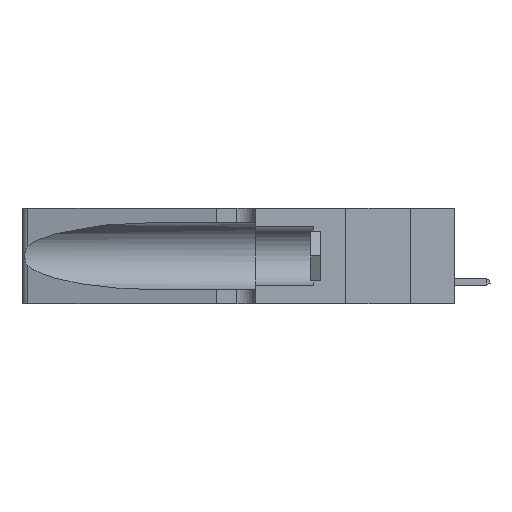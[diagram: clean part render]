
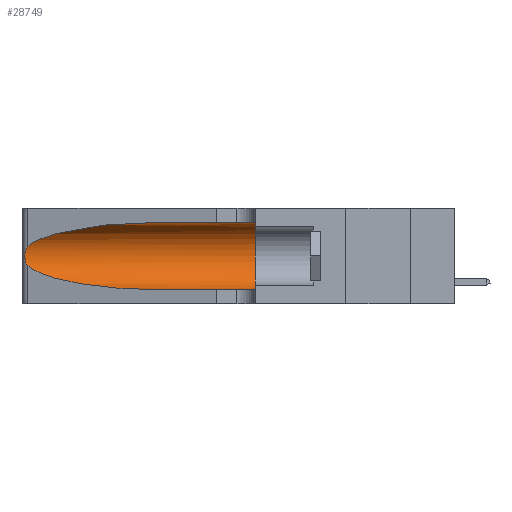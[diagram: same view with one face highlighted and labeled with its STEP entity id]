
A CAD part, left-side view. The second image highlights one B-rep face of the part: STEP entity #28749.
In plain terms, the highlighted cylindrical face has radius 3.308 mm (diameter 6.617 mm), a partial arc.
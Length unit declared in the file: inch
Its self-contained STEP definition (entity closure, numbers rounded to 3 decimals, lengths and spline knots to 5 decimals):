
#87 = EDGE_CURVE ( 'NONE', #42575, #25250, #36162, .T. ) ;
#454 = CARTESIAN_POINT ( 'NONE',  ( 0.26075, 1.23896, 0.19203 ) ) ;
#1236 = CARTESIAN_POINT ( 'NONE',  ( 0.18966, 0.96281, 0.05475 ) ) ;
#2499 = ORIENTED_EDGE ( 'NONE', *, *, #24672, .T. ) ;
#2768 = ORIENTED_EDGE ( 'NONE', *, *, #87, .T. ) ;
#3598 = ORIENTED_EDGE ( 'NONE', *, *, #13376, .T. ) ;
#3885 = CARTESIAN_POINT ( 'NONE',  ( 0.25487, 1.22718, 0.14631 ) ) ;
#4809 = EDGE_CURVE ( 'NONE', #7734, #35645, #37289, .T. ) ;
#5608 = CARTESIAN_POINT ( 'NONE',  ( 0.1305, 0.72297, 0.31525 ) ) ;
#7007 = DIRECTION ( 'NONE',  ( 0., 1., 0. ) ) ;
#7612 = CARTESIAN_POINT ( 'NONE',  ( 0.25555, 1.22993, 0.14849 ) ) ;
#7734 = VERTEX_POINT ( 'NONE', #22920 ) ;
#8442 = AXIS2_PLACEMENT_3D ( 'NONE', #31408, #7007, #25022 ) ;
#9429 = EDGE_CURVE ( 'NONE', #42575, #39204, #37256, .T. ) ;
#9610 = EDGE_LOOP ( 'NONE', ( #2768, #3598, #2499, #30707, #37949, #14089 ) ) ;
#10676 = VECTOR ( 'NONE', #27602, 39.37008 ) ;
#10826 = CARTESIAN_POINT ( 'NONE',  ( 0.1305, 0.35, 0.05475 ) ) ;
#11096 = CARTESIAN_POINT ( 'NONE',  ( 0.25856, 1.23593, 0.16098 ) ) ;
#11572 = CARTESIAN_POINT ( 'NONE',  ( 0.1305, 0.72297, 0.31525 ) ) ;
#12338 = CARTESIAN_POINT ( 'NONE',  ( 0.25487, 1.22718, 0.22369 ) ) ;
#13376 = EDGE_CURVE ( 'NONE', #25250, #31872, #28088, .T. ) ;
#14089 = ORIENTED_EDGE ( 'NONE', *, *, #9429, .F. ) ;
#14602 = CARTESIAN_POINT ( 'NONE',  ( 0.25487, 1.22718, 0.14631 ) ) ;
#14903 = CARTESIAN_POINT ( 'NONE',  ( 0.26075, 1.23896, 0.178 ) ) ;
#15527 = VECTOR ( 'NONE', #39490, 39.37008 ) ;
#16124 = CARTESIAN_POINT ( 'NONE',  ( 0.18966, 0.96281, 0.31525 ) ) ;
#16936 = AXIS2_PLACEMENT_3D ( 'NONE', #19787, #40764, #20544 ) ;
#17925 = CARTESIAN_POINT ( 'NONE',  ( 0.25639, 1.23186, 0.15144 ) ) ;
#18526 = CARTESIAN_POINT ( 'NONE',  ( 0.25487, 1.22718, 0.14631 ) ) ;
#19787 = CARTESIAN_POINT ( 'NONE',  ( 0.1305, 1.61858, 0.185 ) ) ;
#19895 = CARTESIAN_POINT ( 'NONE',  ( 0.2373, 1.15595, 0.28018 ) ) ;
#20544 = DIRECTION ( 'NONE',  ( 0., 0., -1. ) ) ;
#21104 = CARTESIAN_POINT ( 'NONE',  ( 0.26018, 1.23835, 0.19895 ) ) ;
#21437 = CARTESIAN_POINT ( 'NONE',  ( 0.1305, 0.72297, 0.05475 ) ) ;
#22044 = CARTESIAN_POINT ( 'NONE',  ( 0.2373, 1.15595, 0.08982 ) ) ;
#22920 = CARTESIAN_POINT ( 'NONE',  ( 0.1305, 0.72297, 0.05475 ) ) ;
#24672 = EDGE_CURVE ( 'NONE', #31872, #7734, #29031, .T. ) ;
#25022 = DIRECTION ( 'NONE',  ( 0., 0., 1. ) ) ;
#25059 = CARTESIAN_POINT ( 'NONE',  ( 0.25639, 1.23184, 0.21858 ) ) ;
#25192 = CARTESIAN_POINT ( 'NONE',  ( 0.1305, 1.61858, 0.31525 ) ) ;
#25250 = VERTEX_POINT ( 'NONE', #43788 ) ;
#26357 = CIRCLE ( 'NONE', #8442, 0.13025 ) ;
#26851 = CYLINDRICAL_SURFACE ( 'NONE', #16936, 0.13025 ) ;
#27602 = DIRECTION ( 'NONE',  ( 0., -1., 0. ) ) ;
#28088 = B_SPLINE_CURVE_WITH_KNOTS ( 'NONE', 3,
 ( #39044, #32179, #25059, #39203, #35658, #21104, #454, #14903, #35217, #11096, #38742, #17925, #7612, #14602 ),
 .UNSPECIFIED., .F., .F.,
 ( 4, 2, 2, 2, 2, 2, 4 ),
 ( 0., 0.00027, 0.00053, 0.00107, 0.0016, 0.00187, 0.00214 ),
 .UNSPECIFIED. ) ;
#28749 = ADVANCED_FACE ( 'NONE', ( #38255 ), #26851, .F. ) ;
#29031 =( BOUNDED_CURVE ( )  B_SPLINE_CURVE ( 3, ( #18526, #22044, #1236, #21437 ),
 .UNSPECIFIED., .F., .F. ) 
 B_SPLINE_CURVE_WITH_KNOTS ( ( 4, 4 ),
 ( 3.44316, 4.71239 ),
 .UNSPECIFIED. ) 
 CURVE ( )  GEOMETRIC_REPRESENTATION_ITEM ( )  RATIONAL_B_SPLINE_CURVE ( ( 1., 0.87, 0.87, 1. ) ) 
 REPRESENTATION_ITEM ( '' )  );
#30707 = ORIENTED_EDGE ( 'NONE', *, *, #4809, .T. ) ;
#31408 = CARTESIAN_POINT ( 'NONE',  ( 0.1305, 0.35, 0.185 ) ) ;
#31872 = VERTEX_POINT ( 'NONE', #3885 ) ;
#32179 = CARTESIAN_POINT ( 'NONE',  ( 0.25555, 1.22994, 0.2215 ) ) ;
#35217 = CARTESIAN_POINT ( 'NONE',  ( 0.26017, 1.23833, 0.17102 ) ) ;
#35645 = VERTEX_POINT ( 'NONE', #10826 ) ;
#35658 = CARTESIAN_POINT ( 'NONE',  ( 0.25854, 1.2359, 0.20912 ) ) ;
#36162 =( BOUNDED_CURVE ( )  B_SPLINE_CURVE ( 3, ( #5608, #16124, #19895, #12338 ),
 .UNSPECIFIED., .F., .F. ) 
 B_SPLINE_CURVE_WITH_KNOTS ( ( 4, 4 ),
 ( 1.5708, 2.84003 ),
 .UNSPECIFIED. ) 
 CURVE ( )  GEOMETRIC_REPRESENTATION_ITEM ( )  RATIONAL_B_SPLINE_CURVE ( ( 1., 0.87, 0.87, 1. ) ) 
 REPRESENTATION_ITEM ( '' )  );
#37256 = LINE ( 'NONE', #25192, #15527 ) ;
#37289 = LINE ( 'NONE', #37797, #10676 ) ;
#37797 = CARTESIAN_POINT ( 'NONE',  ( 0.1305, 1.61858, 0.05475 ) ) ;
#37949 = ORIENTED_EDGE ( 'NONE', *, *, #40084, .F. ) ;
#38255 = FACE_OUTER_BOUND ( 'NONE', #9610, .T. ) ;
#38742 = CARTESIAN_POINT ( 'NONE',  ( 0.25789, 1.23486, 0.15765 ) ) ;
#39044 = CARTESIAN_POINT ( 'NONE',  ( 0.25487, 1.22718, 0.22369 ) ) ;
#39203 = CARTESIAN_POINT ( 'NONE',  ( 0.25787, 1.23484, 0.2124 ) ) ;
#39204 = VERTEX_POINT ( 'NONE', #43442 ) ;
#39490 = DIRECTION ( 'NONE',  ( 0., -1., 0. ) ) ;
#40084 = EDGE_CURVE ( 'NONE', #39204, #35645, #26357, .T. ) ;
#40764 = DIRECTION ( 'NONE',  ( 0., -1., 0. ) ) ;
#42575 = VERTEX_POINT ( 'NONE', #11572 ) ;
#43442 = CARTESIAN_POINT ( 'NONE',  ( 0.1305, 0.35, 0.31525 ) ) ;
#43788 = CARTESIAN_POINT ( 'NONE',  ( 0.25487, 1.22718, 0.22369 ) ) ;
